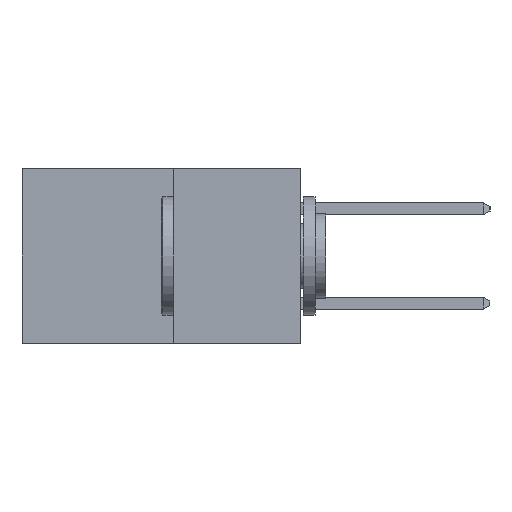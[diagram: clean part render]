
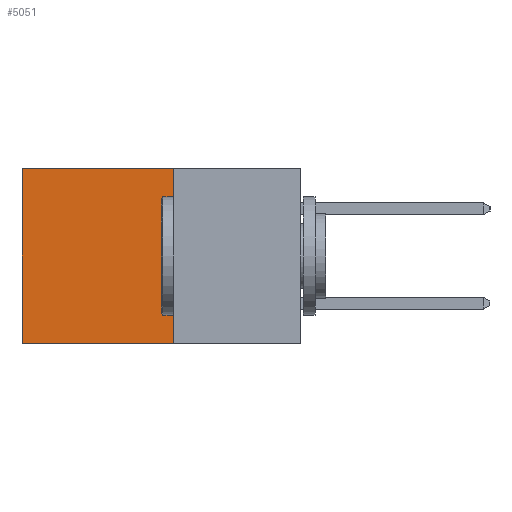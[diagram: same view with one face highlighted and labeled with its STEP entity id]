
A CAD part, left-side view. The second image highlights one B-rep face of the part: STEP entity #5051.
In plain terms, the highlighted planar face has unit normal (-1, 0, 0).
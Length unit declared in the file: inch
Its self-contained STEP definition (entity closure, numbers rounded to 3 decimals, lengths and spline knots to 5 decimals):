
#305 = VERTEX_POINT ( 'NONE', #4077 ) ;
#547 = EDGE_CURVE ( 'NONE', #2005, #1268, #8225, .T. ) ;
#870 = CARTESIAN_POINT ( 'NONE',  ( 0.277, 0.27, -0.37 ) ) ;
#889 = EDGE_CURVE ( 'NONE', #305, #2005, #5075, .T. ) ;
#1197 = VECTOR ( 'NONE', #9515, 39.37008 ) ;
#1207 = DIRECTION ( 'NONE',  ( 0., 1., 0. ) ) ;
#1268 = VERTEX_POINT ( 'NONE', #1995 ) ;
#1504 = ORIENTED_EDGE ( 'NONE', *, *, #547, .T. ) ;
#1665 = ORIENTED_EDGE ( 'NONE', *, *, #889, .T. ) ;
#1995 = CARTESIAN_POINT ( 'NONE',  ( 0.277, 0.59, -0.37 ) ) ;
#1996 = EDGE_CURVE ( 'NONE', #10251, #1268, #10348, .T. ) ;
#2005 = VERTEX_POINT ( 'NONE', #4347 ) ;
#2452 = CARTESIAN_POINT ( 'NONE',  ( 0.277, 0.27, -0.37 ) ) ;
#2502 = LINE ( 'NONE', #870, #8783 ) ;
#2845 = CARTESIAN_POINT ( 'NONE',  ( 0.277, 0.27, 0. ) ) ;
#2971 = EDGE_LOOP ( 'NONE', ( #1504, #4538, #9225, #1665 ) ) ;
#2979 = VECTOR ( 'NONE', #1207, 39.37008 ) ;
#3024 = EDGE_CURVE ( 'NONE', #305, #10251, #2502, .T. ) ;
#3090 = DIRECTION ( 'NONE',  ( 0., 0., -1. ) ) ;
#4077 = CARTESIAN_POINT ( 'NONE',  ( 0.277, 0.27, 0. ) ) ;
#4183 = AXIS2_PLACEMENT_3D ( 'NONE', #10342, #10280, #10272 ) ;
#4347 = CARTESIAN_POINT ( 'NONE',  ( 0.277, 0.59, 0. ) ) ;
#4538 = ORIENTED_EDGE ( 'NONE', *, *, #1996, .F. ) ;
#5051 = ADVANCED_FACE ( 'NONE', ( #7103 ), #10291, .F. ) ;
#5075 = LINE ( 'NONE', #2845, #2979 ) ;
#6294 = DIRECTION ( 'NONE',  ( 0., 0., -1. ) ) ;
#6304 = CARTESIAN_POINT ( 'NONE',  ( 0.277, 0.59, -0.37 ) ) ;
#7103 = FACE_OUTER_BOUND ( 'NONE', #2971, .T. ) ;
#7996 = CARTESIAN_POINT ( 'NONE',  ( 0.277, 0.27, -0.37 ) ) ;
#8225 = LINE ( 'NONE', #6304, #10651 ) ;
#8783 = VECTOR ( 'NONE', #3090, 39.37008 ) ;
#9225 = ORIENTED_EDGE ( 'NONE', *, *, #3024, .F. ) ;
#9515 = DIRECTION ( 'NONE',  ( 0., 1., 0. ) ) ;
#10251 = VERTEX_POINT ( 'NONE', #7996 ) ;
#10272 = DIRECTION ( 'NONE',  ( 0., 0., -1. ) ) ;
#10280 = DIRECTION ( 'NONE',  ( 1., 0., 0. ) ) ;
#10291 = PLANE ( 'NONE',  #4183 ) ;
#10342 = CARTESIAN_POINT ( 'NONE',  ( 0.277, 0.27, -0.37 ) ) ;
#10348 = LINE ( 'NONE', #2452, #1197 ) ;
#10651 = VECTOR ( 'NONE', #6294, 39.37008 ) ;
